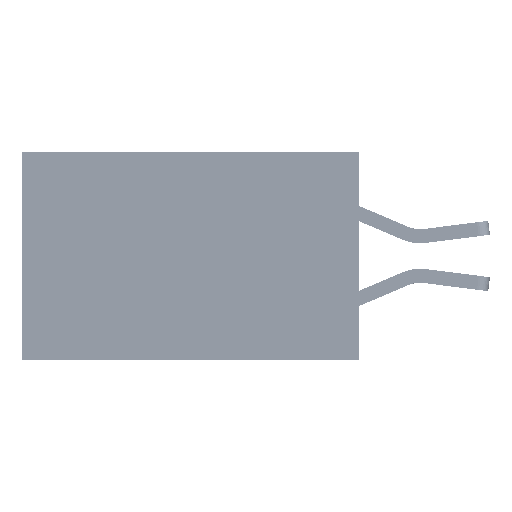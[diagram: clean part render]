
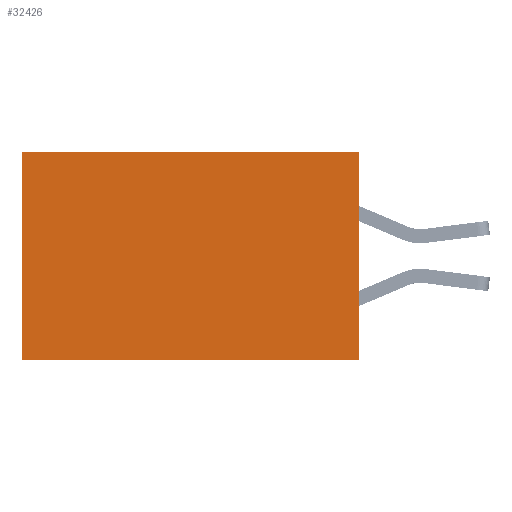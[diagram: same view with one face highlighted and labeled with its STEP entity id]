
A CAD part, left-side view. The second image highlights one B-rep face of the part: STEP entity #32426.
In plain terms, the highlighted planar face has unit normal (-1, 0, 0).
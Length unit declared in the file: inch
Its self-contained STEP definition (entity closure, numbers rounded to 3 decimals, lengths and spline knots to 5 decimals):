
#46 = DIRECTION ( 'NONE',  ( 0., 1., 0. ) ) ;
#470 = DIRECTION ( 'NONE',  ( 0., 0., -1. ) ) ;
#1563 = DIRECTION ( 'NONE',  ( 0., 1., 0. ) ) ;
#1744 = DIRECTION ( 'NONE',  ( 1., 0., 0. ) ) ;
#2683 = ORIENTED_EDGE ( 'NONE', *, *, #5859, .F. ) ;
#3115 = FACE_OUTER_BOUND ( 'NONE', #30241, .T. ) ;
#3869 = CARTESIAN_POINT ( 'NONE',  ( 0.2875, 0.6, -0.37 ) ) ;
#4625 = VERTEX_POINT ( 'NONE', #3869 ) ;
#5859 = EDGE_CURVE ( 'NONE', #9804, #6950, #29298, .T. ) ;
#6658 = DIRECTION ( 'NONE',  ( 0., 0., -1. ) ) ;
#6950 = VERTEX_POINT ( 'NONE', #13568 ) ;
#7100 = LINE ( 'NONE', #9974, #38662 ) ;
#7646 = CARTESIAN_POINT ( 'NONE',  ( 0.2875, 0., 0. ) ) ;
#7734 = VECTOR ( 'NONE', #46, 39.37008 ) ;
#8718 = ORIENTED_EDGE ( 'NONE', *, *, #20224, .F. ) ;
#9804 = VERTEX_POINT ( 'NONE', #7646 ) ;
#9974 = CARTESIAN_POINT ( 'NONE',  ( 0.2875, 0.6, 0. ) ) ;
#12144 = CARTESIAN_POINT ( 'NONE',  ( 0.2875, 0., -0.37 ) ) ;
#12162 = CARTESIAN_POINT ( 'NONE',  ( 0.2875, 0., 0. ) ) ;
#12297 = VECTOR ( 'NONE', #1563, 39.37008 ) ;
#13568 = CARTESIAN_POINT ( 'NONE',  ( 0.2875, 0., -0.37 ) ) ;
#15439 = EDGE_CURVE ( 'NONE', #20097, #4625, #7100, .T. ) ;
#16616 = LINE ( 'NONE', #25891, #12297 ) ;
#18190 = ORIENTED_EDGE ( 'NONE', *, *, #15439, .T. ) ;
#18799 = VECTOR ( 'NONE', #470, 39.37008 ) ;
#19514 = PLANE ( 'NONE',  #35206 ) ;
#19733 = LINE ( 'NONE', #12144, #7734 ) ;
#20097 = VERTEX_POINT ( 'NONE', #32894 ) ;
#20224 = EDGE_CURVE ( 'NONE', #6950, #4625, #19733, .T. ) ;
#23007 = ORIENTED_EDGE ( 'NONE', *, *, #28106, .T. ) ;
#25891 = CARTESIAN_POINT ( 'NONE',  ( 0.2875, 0., 0. ) ) ;
#28106 = EDGE_CURVE ( 'NONE', #9804, #20097, #16616, .T. ) ;
#28999 = DIRECTION ( 'NONE',  ( 0., 0., -1. ) ) ;
#29298 = LINE ( 'NONE', #12162, #18799 ) ;
#30241 = EDGE_LOOP ( 'NONE', ( #18190, #8718, #2683, #23007 ) ) ;
#32315 = CARTESIAN_POINT ( 'NONE',  ( 0.2875, 0., 0. ) ) ;
#32426 = ADVANCED_FACE ( 'NONE', ( #3115 ), #19514, .F. ) ;
#32894 = CARTESIAN_POINT ( 'NONE',  ( 0.2875, 0.6, 0. ) ) ;
#35206 = AXIS2_PLACEMENT_3D ( 'NONE', #32315, #1744, #28999 ) ;
#38662 = VECTOR ( 'NONE', #6658, 39.37008 ) ;
